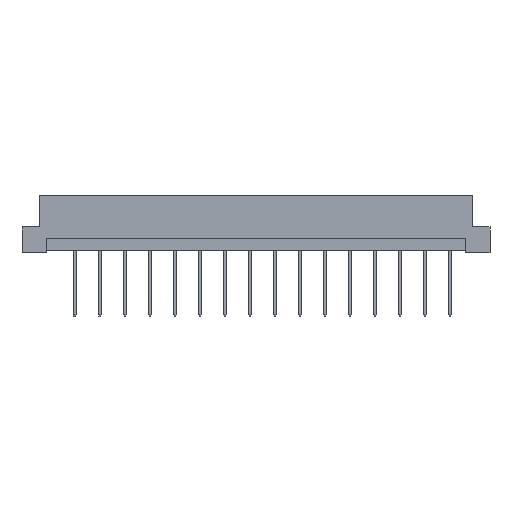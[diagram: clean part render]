
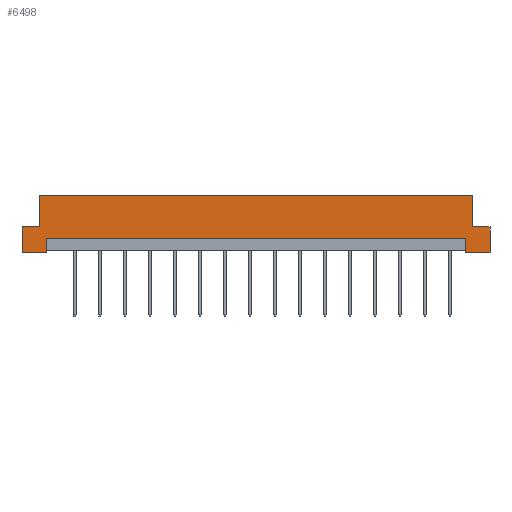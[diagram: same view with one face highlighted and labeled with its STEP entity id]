
A CAD part, front view. The second image highlights one B-rep face of the part: STEP entity #6498.
In plain terms, the highlighted planar face has unit normal (0, -1, 0).
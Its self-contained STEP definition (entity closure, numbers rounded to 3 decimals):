
#263 = EDGE_CURVE ( 'NONE', #6875, #16594, #4320, .T. ) ;
#330 = DIRECTION ( 'NONE',  ( -1., 0., 0. ) ) ;
#453 = AXIS2_PLACEMENT_3D ( 'NONE', #8857, #10135, #12627 ) ;
#497 = LINE ( 'NONE', #13256, #13325 ) ;
#800 = CARTESIAN_POINT ( 'NONE',  ( 44., 0., 5.2 ) ) ;
#1020 = ORIENTED_EDGE ( 'NONE', *, *, #6714, .F. ) ;
#1089 = CARTESIAN_POINT ( 'NONE',  ( 44., 0., 5.2 ) ) ;
#1473 = DIRECTION ( 'NONE',  ( 0., 0., 1. ) ) ;
#1532 = DIRECTION ( 'NONE',  ( 0., 0., -1. ) ) ;
#1763 = CARTESIAN_POINT ( 'NONE',  ( -42.6, 0., 0. ) ) ;
#1775 = VERTEX_POINT ( 'NONE', #1089 ) ;
#2062 = EDGE_CURVE ( 'NONE', #14420, #15152, #497, .T. ) ;
#2485 = CARTESIAN_POINT ( 'NONE',  ( -47.5, 0., 0. ) ) ;
#2528 = DIRECTION ( 'NONE',  ( 0., 0., 1. ) ) ;
#2563 = EDGE_CURVE ( 'NONE', #10841, #3960, #2715, .T. ) ;
#2715 = LINE ( 'NONE', #13070, #12461 ) ;
#2785 = ORIENTED_EDGE ( 'NONE', *, *, #7673, .F. ) ;
#3133 = DIRECTION ( 'NONE',  ( 0., 0., -1. ) ) ;
#3144 = VERTEX_POINT ( 'NONE', #4879 ) ;
#3162 = VECTOR ( 'NONE', #8878, 1000. ) ;
#3232 = VERTEX_POINT ( 'NONE', #2485 ) ;
#3452 = DIRECTION ( 'NONE',  ( 0., 0., 1. ) ) ;
#3816 = EDGE_CURVE ( 'NONE', #9637, #10841, #4945, .T. ) ;
#3908 = ORIENTED_EDGE ( 'NONE', *, *, #3816, .F. ) ;
#3960 = VERTEX_POINT ( 'NONE', #1763 ) ;
#3986 = CARTESIAN_POINT ( 'NONE',  ( -47.5, 0., 11.6 ) ) ;
#4037 = CARTESIAN_POINT ( 'NONE',  ( -44., 0., 11.6 ) ) ;
#4137 = LINE ( 'NONE', #8169, #4289 ) ;
#4289 = VECTOR ( 'NONE', #14499, 1000. ) ;
#4320 = LINE ( 'NONE', #3986, #11163 ) ;
#4609 = ORIENTED_EDGE ( 'NONE', *, *, #8275, .F. ) ;
#4879 = CARTESIAN_POINT ( 'NONE',  ( -47.5, 0., 5.2 ) ) ;
#4920 = PLANE ( 'NONE',  #453 ) ;
#4945 = LINE ( 'NONE', #12907, #3162 ) ;
#5001 = CARTESIAN_POINT ( 'NONE',  ( -42.6, 0., 2.9 ) ) ;
#5018 = ORIENTED_EDGE ( 'NONE', *, *, #2062, .F. ) ;
#5172 = LINE ( 'NONE', #16719, #7649 ) ;
#5432 = LINE ( 'NONE', #14507, #5962 ) ;
#5619 = VECTOR ( 'NONE', #14002, 1000. ) ;
#5763 = EDGE_CURVE ( 'NONE', #1775, #7367, #5432, .T. ) ;
#5962 = VECTOR ( 'NONE', #8087, 1000. ) ;
#5977 = EDGE_CURVE ( 'NONE', #1775, #16594, #15085, .T. ) ;
#6444 = ORIENTED_EDGE ( 'NONE', *, *, #9567, .F. ) ;
#6478 = VECTOR ( 'NONE', #1473, 1000. ) ;
#6498 = ADVANCED_FACE ( 'NONE', ( #16716 ), #4920, .F. ) ;
#6714 = EDGE_CURVE ( 'NONE', #3960, #3232, #4137, .T. ) ;
#6875 = VERTEX_POINT ( 'NONE', #4037 ) ;
#6978 = LINE ( 'NONE', #14853, #11016 ) ;
#7255 = EDGE_CURVE ( 'NONE', #7367, #14420, #10184, .T. ) ;
#7263 = ORIENTED_EDGE ( 'NONE', *, *, #13363, .T. ) ;
#7367 = VERTEX_POINT ( 'NONE', #7783 ) ;
#7466 = ORIENTED_EDGE ( 'NONE', *, *, #5977, .T. ) ;
#7649 = VECTOR ( 'NONE', #2528, 1000. ) ;
#7673 = EDGE_CURVE ( 'NONE', #8234, #6875, #5172, .T. ) ;
#7783 = CARTESIAN_POINT ( 'NONE',  ( 47.5, 0., 5.2 ) ) ;
#8087 = DIRECTION ( 'NONE',  ( 1., 0., 0. ) ) ;
#8151 = CARTESIAN_POINT ( 'NONE',  ( -44., 0., 5.2 ) ) ;
#8169 = CARTESIAN_POINT ( 'NONE',  ( -47.5, 0., 0. ) ) ;
#8234 = VERTEX_POINT ( 'NONE', #8151 ) ;
#8270 = ORIENTED_EDGE ( 'NONE', *, *, #263, .F. ) ;
#8275 = EDGE_CURVE ( 'NONE', #3232, #3144, #10711, .T. ) ;
#8772 = CARTESIAN_POINT ( 'NONE',  ( -47.5, 0., 5.2 ) ) ;
#8857 = CARTESIAN_POINT ( 'NONE',  ( -47.5, 0., 11.6 ) ) ;
#8878 = DIRECTION ( 'NONE',  ( -1., 0., 0. ) ) ;
#8895 = CARTESIAN_POINT ( 'NONE',  ( 47.5, 0., 0. ) ) ;
#9027 = VECTOR ( 'NONE', #1532, 1000. ) ;
#9138 = ORIENTED_EDGE ( 'NONE', *, *, #5763, .F. ) ;
#9567 = EDGE_CURVE ( 'NONE', #3144, #8234, #11171, .T. ) ;
#9637 = VERTEX_POINT ( 'NONE', #14480 ) ;
#10135 = DIRECTION ( 'NONE',  ( 0., 1., 0. ) ) ;
#10184 = LINE ( 'NONE', #8895, #9027 ) ;
#10711 = LINE ( 'NONE', #14391, #6478 ) ;
#10841 = VERTEX_POINT ( 'NONE', #5001 ) ;
#11016 = VECTOR ( 'NONE', #3133, 1000. ) ;
#11163 = VECTOR ( 'NONE', #14762, 1000. ) ;
#11171 = LINE ( 'NONE', #8772, #5619 ) ;
#12328 = CARTESIAN_POINT ( 'NONE',  ( 47.5, 0., 0. ) ) ;
#12461 = VECTOR ( 'NONE', #14522, 1000. ) ;
#12627 = DIRECTION ( 'NONE',  ( 0., 0., 1. ) ) ;
#12907 = CARTESIAN_POINT ( 'NONE',  ( 42.6, 0., 2.9 ) ) ;
#13070 = CARTESIAN_POINT ( 'NONE',  ( -42.6, 0., 0.5 ) ) ;
#13256 = CARTESIAN_POINT ( 'NONE',  ( -47.5, 0., 0. ) ) ;
#13325 = VECTOR ( 'NONE', #330, 1000. ) ;
#13363 = EDGE_CURVE ( 'NONE', #9637, #15152, #6978, .T. ) ;
#13562 = ORIENTED_EDGE ( 'NONE', *, *, #2563, .F. ) ;
#13882 = CARTESIAN_POINT ( 'NONE',  ( 44., 0., 11.6 ) ) ;
#14002 = DIRECTION ( 'NONE',  ( 1., 0., 0. ) ) ;
#14391 = CARTESIAN_POINT ( 'NONE',  ( -47.5, 0., 0. ) ) ;
#14420 = VERTEX_POINT ( 'NONE', #12328 ) ;
#14480 = CARTESIAN_POINT ( 'NONE',  ( 42.6, 0., 2.9 ) ) ;
#14499 = DIRECTION ( 'NONE',  ( -1., 0., 0. ) ) ;
#14507 = CARTESIAN_POINT ( 'NONE',  ( 47.5, 0., 5.2 ) ) ;
#14522 = DIRECTION ( 'NONE',  ( 0., 0., -1. ) ) ;
#14762 = DIRECTION ( 'NONE',  ( 1., 0., 0. ) ) ;
#14853 = CARTESIAN_POINT ( 'NONE',  ( 42.6, 0., 0.5 ) ) ;
#14993 = ORIENTED_EDGE ( 'NONE', *, *, #7255, .F. ) ;
#15085 = LINE ( 'NONE', #800, #15528 ) ;
#15152 = VERTEX_POINT ( 'NONE', #15677 ) ;
#15194 = EDGE_LOOP ( 'NONE', ( #3908, #7263, #5018, #14993, #9138, #7466, #8270, #2785, #6444, #4609, #1020, #13562 ) ) ;
#15528 = VECTOR ( 'NONE', #3452, 1000. ) ;
#15677 = CARTESIAN_POINT ( 'NONE',  ( 42.6, 0., 0. ) ) ;
#16594 = VERTEX_POINT ( 'NONE', #13882 ) ;
#16716 = FACE_OUTER_BOUND ( 'NONE', #15194, .T. ) ;
#16719 = CARTESIAN_POINT ( 'NONE',  ( -44., 0., 5.2 ) ) ;
